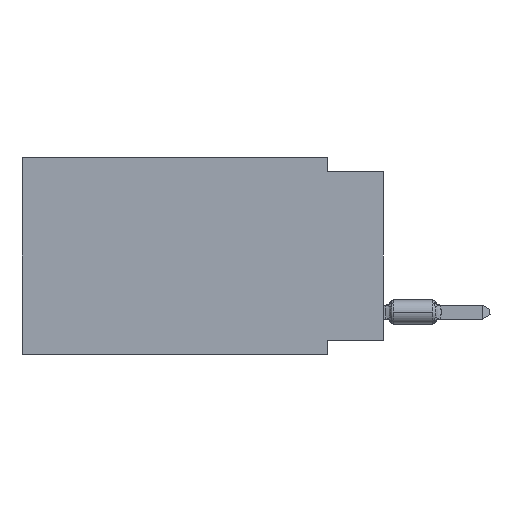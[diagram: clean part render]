
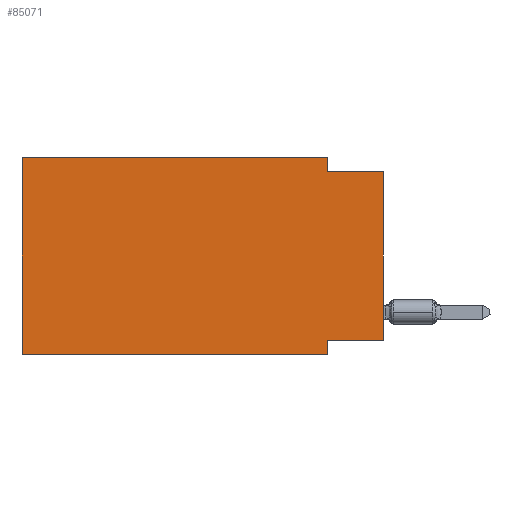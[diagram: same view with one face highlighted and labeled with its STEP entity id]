
A CAD part, left-side view. The second image highlights one B-rep face of the part: STEP entity #85071.
In plain terms, the highlighted planar face has unit normal (-1, 0, 0).
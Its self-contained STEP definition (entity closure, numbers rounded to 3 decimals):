
#704 = VECTOR ( 'NONE', #36759, 1000. ) ;
#904 = VECTOR ( 'NONE', #12249, 1000. ) ;
#1356 = CARTESIAN_POINT ( 'NONE',  ( 0., 16.383, 0. ) ) ;
#3671 = EDGE_CURVE ( 'NONE', #17318, #49447, #62639, .T. ) ;
#6381 = CARTESIAN_POINT ( 'NONE',  ( 0., 0., 0. ) ) ;
#7147 = ORIENTED_EDGE ( 'NONE', *, *, #48509, .F. ) ;
#7325 = DIRECTION ( 'NONE',  ( 1., 0., 0. ) ) ;
#9440 = EDGE_CURVE ( 'NONE', #22629, #94134, #74369, .T. ) ;
#9645 = CARTESIAN_POINT ( 'NONE',  ( 0., 0., -0.635 ) ) ;
#11186 = CARTESIAN_POINT ( 'NONE',  ( 0., 2.54, -8.255 ) ) ;
#12249 = DIRECTION ( 'NONE',  ( 0., 0., 1. ) ) ;
#15830 = LINE ( 'NONE', #55015, #79145 ) ;
#17318 = VERTEX_POINT ( 'NONE', #67360 ) ;
#18139 = ORIENTED_EDGE ( 'NONE', *, *, #3671, .T. ) ;
#19608 = VECTOR ( 'NONE', #66921, 1000. ) ;
#19676 = CARTESIAN_POINT ( 'NONE',  ( 0., 16.383, 0. ) ) ;
#22629 = VERTEX_POINT ( 'NONE', #84570 ) ;
#23744 = DIRECTION ( 'NONE',  ( 0., 0., -1. ) ) ;
#25615 = VECTOR ( 'NONE', #42260, 1000. ) ;
#26559 = CARTESIAN_POINT ( 'NONE',  ( 0., 2.54, -0.635 ) ) ;
#26782 = VERTEX_POINT ( 'NONE', #26559 ) ;
#32362 = CARTESIAN_POINT ( 'NONE',  ( 0., 16.383, -8.89 ) ) ;
#34416 = ORIENTED_EDGE ( 'NONE', *, *, #73543, .F. ) ;
#35263 = VERTEX_POINT ( 'NONE', #11186 ) ;
#36759 = DIRECTION ( 'NONE',  ( 0., -1., 0. ) ) ;
#36916 = VERTEX_POINT ( 'NONE', #40041 ) ;
#38727 = DIRECTION ( 'NONE',  ( 0., -1., 0. ) ) ;
#40041 = CARTESIAN_POINT ( 'NONE',  ( 0., 2.54, 0. ) ) ;
#40766 = DIRECTION ( 'NONE',  ( 0., -1., 0. ) ) ;
#41363 = LINE ( 'NONE', #87527, #58204 ) ;
#42260 = DIRECTION ( 'NONE',  ( 0., 0., -1. ) ) ;
#44225 = CARTESIAN_POINT ( 'NONE',  ( 0., 2.54, 0. ) ) ;
#46218 = EDGE_CURVE ( 'NONE', #17318, #87956, #87703, .T. ) ;
#46440 = ORIENTED_EDGE ( 'NONE', *, *, #9440, .T. ) ;
#46631 = LINE ( 'NONE', #68513, #704 ) ;
#48509 = EDGE_CURVE ( 'NONE', #22629, #35263, #41363, .T. ) ;
#49447 = VERTEX_POINT ( 'NONE', #75195 ) ;
#51503 = CARTESIAN_POINT ( 'NONE',  ( 0., 16.383, 0. ) ) ;
#52005 = DIRECTION ( 'NONE',  ( 0., 0., -1. ) ) ;
#55015 = CARTESIAN_POINT ( 'NONE',  ( 0., 2.54, -8.89 ) ) ;
#58060 = VECTOR ( 'NONE', #38727, 1000. ) ;
#58204 = VECTOR ( 'NONE', #71653, 1000. ) ;
#58899 = EDGE_CURVE ( 'NONE', #26782, #94134, #83939, .T. ) ;
#59118 = LINE ( 'NONE', #44225, #25615 ) ;
#60903 = PLANE ( 'NONE',  #73623 ) ;
#61132 = VECTOR ( 'NONE', #40766, 1000. ) ;
#62639 = LINE ( 'NONE', #32362, #61132 ) ;
#64450 = ORIENTED_EDGE ( 'NONE', *, *, #58899, .F. ) ;
#65024 = ORIENTED_EDGE ( 'NONE', *, *, #46218, .F. ) ;
#65900 = EDGE_CURVE ( 'NONE', #35263, #49447, #15830, .T. ) ;
#66921 = DIRECTION ( 'NONE',  ( 0., 0., 1. ) ) ;
#67360 = CARTESIAN_POINT ( 'NONE',  ( 0., 16.383, -8.89 ) ) ;
#68513 = CARTESIAN_POINT ( 'NONE',  ( 0., 16.383, 0. ) ) ;
#71653 = DIRECTION ( 'NONE',  ( 0., 1., 0. ) ) ;
#73151 = ORIENTED_EDGE ( 'NONE', *, *, #76750, .F. ) ;
#73543 = EDGE_CURVE ( 'NONE', #36916, #26782, #59118, .T. ) ;
#73623 = AXIS2_PLACEMENT_3D ( 'NONE', #51503, #7325, #52005 ) ;
#74369 = LINE ( 'NONE', #6381, #19608 ) ;
#75195 = CARTESIAN_POINT ( 'NONE',  ( 0., 2.54, -8.89 ) ) ;
#76750 = EDGE_CURVE ( 'NONE', #87956, #36916, #46631, .T. ) ;
#77233 = EDGE_LOOP ( 'NONE', ( #46440, #64450, #34416, #73151, #65024, #18139, #78915, #7147 ) ) ;
#78915 = ORIENTED_EDGE ( 'NONE', *, *, #65900, .F. ) ;
#79145 = VECTOR ( 'NONE', #23744, 1000. ) ;
#81312 = FACE_OUTER_BOUND ( 'NONE', #77233, .T. ) ;
#83939 = LINE ( 'NONE', #91386, #58060 ) ;
#84570 = CARTESIAN_POINT ( 'NONE',  ( 0., 0., -8.255 ) ) ;
#85071 = ADVANCED_FACE ( 'NONE', ( #81312 ), #60903, .F. ) ;
#87527 = CARTESIAN_POINT ( 'NONE',  ( 0., 0., -8.255 ) ) ;
#87703 = LINE ( 'NONE', #19676, #904 ) ;
#87956 = VERTEX_POINT ( 'NONE', #1356 ) ;
#91386 = CARTESIAN_POINT ( 'NONE',  ( 0., 0., -0.635 ) ) ;
#94134 = VERTEX_POINT ( 'NONE', #9645 ) ;
